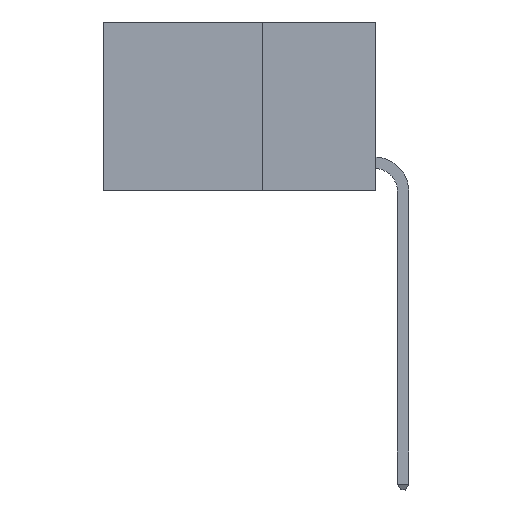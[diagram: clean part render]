
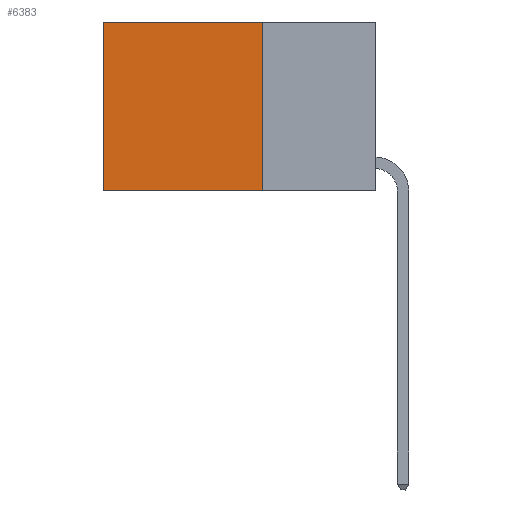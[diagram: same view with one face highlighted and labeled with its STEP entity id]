
A CAD part, left-side view. The second image highlights one B-rep face of the part: STEP entity #6383.
In plain terms, the highlighted planar face has unit normal (-1, 0, 0).
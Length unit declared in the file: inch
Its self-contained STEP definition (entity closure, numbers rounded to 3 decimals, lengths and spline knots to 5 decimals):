
#84 = ORIENTED_EDGE ( 'NONE', *, *, #1062, .F. ) ;
#931 = FACE_OUTER_BOUND ( 'NONE', #8285, .T. ) ;
#1062 = EDGE_CURVE ( 'NONE', #4363, #9212, #9291, .T. ) ;
#1390 = VERTEX_POINT ( 'NONE', #3964 ) ;
#1546 = EDGE_CURVE ( 'NONE', #4363, #1390, #8707, .T. ) ;
#1710 = DIRECTION ( 'NONE',  ( 0., 1., 0. ) ) ;
#1936 = EDGE_CURVE ( 'NONE', #9212, #9380, #10346, .T. ) ;
#2142 = CARTESIAN_POINT ( 'NONE',  ( 0.2625, 0.6, -0.37 ) ) ;
#2512 = ORIENTED_EDGE ( 'NONE', *, *, #6007, .T. ) ;
#3319 = DIRECTION ( 'NONE',  ( 0., 0., -1. ) ) ;
#3397 = VECTOR ( 'NONE', #3319, 39.37008 ) ;
#3956 = DIRECTION ( 'NONE',  ( 1., 0., 0. ) ) ;
#3964 = CARTESIAN_POINT ( 'NONE',  ( 0.2625, 0.6, 0. ) ) ;
#3983 = CARTESIAN_POINT ( 'NONE',  ( 0.2625, 0.25, 0. ) ) ;
#4363 = VERTEX_POINT ( 'NONE', #10305 ) ;
#4671 = DIRECTION ( 'NONE',  ( 0., 1., 0. ) ) ;
#5334 = VECTOR ( 'NONE', #4671, 39.37008 ) ;
#6007 = EDGE_CURVE ( 'NONE', #1390, #9380, #13172, .T. ) ;
#6148 = AXIS2_PLACEMENT_3D ( 'NONE', #7101, #3956, #11228 ) ;
#6383 = ADVANCED_FACE ( 'NONE', ( #931 ), #10217, .F. ) ;
#7101 = CARTESIAN_POINT ( 'NONE',  ( 0.2625, 0.25, 0. ) ) ;
#7600 = VECTOR ( 'NONE', #1710, 39.37008 ) ;
#7897 = CARTESIAN_POINT ( 'NONE',  ( 0.2625, 0.25, -0.37 ) ) ;
#8285 = EDGE_LOOP ( 'NONE', ( #2512, #9618, #84, #12117 ) ) ;
#8707 = LINE ( 'NONE', #3983, #5334 ) ;
#8985 = DIRECTION ( 'NONE',  ( 0., 0., -1. ) ) ;
#9130 = CARTESIAN_POINT ( 'NONE',  ( 0.2625, 0.25, -0.37 ) ) ;
#9212 = VERTEX_POINT ( 'NONE', #9130 ) ;
#9291 = LINE ( 'NONE', #12508, #3397 ) ;
#9380 = VERTEX_POINT ( 'NONE', #2142 ) ;
#9618 = ORIENTED_EDGE ( 'NONE', *, *, #1936, .F. ) ;
#9887 = VECTOR ( 'NONE', #8985, 39.37008 ) ;
#10217 = PLANE ( 'NONE',  #6148 ) ;
#10305 = CARTESIAN_POINT ( 'NONE',  ( 0.2625, 0.25, 0. ) ) ;
#10346 = LINE ( 'NONE', #7897, #7600 ) ;
#11228 = DIRECTION ( 'NONE',  ( 0., 0., -1. ) ) ;
#12003 = CARTESIAN_POINT ( 'NONE',  ( 0.2625, 0.6, 0. ) ) ;
#12117 = ORIENTED_EDGE ( 'NONE', *, *, #1546, .T. ) ;
#12508 = CARTESIAN_POINT ( 'NONE',  ( 0.2625, 0.25, 0. ) ) ;
#13172 = LINE ( 'NONE', #12003, #9887 ) ;
